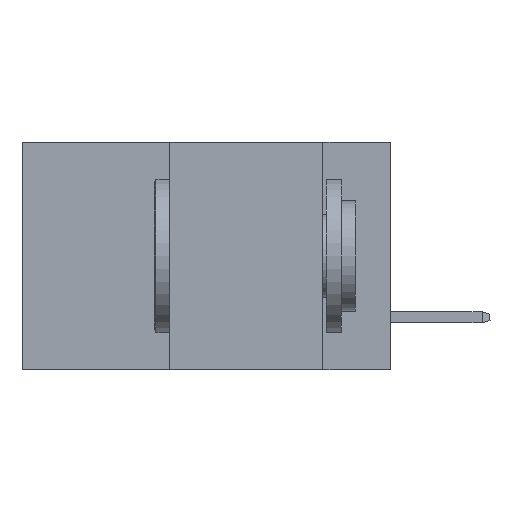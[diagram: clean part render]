
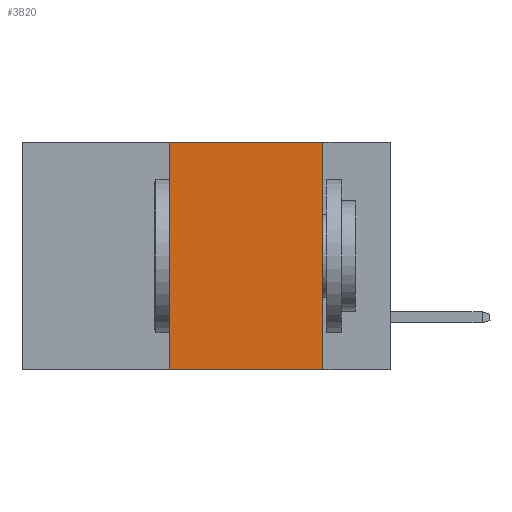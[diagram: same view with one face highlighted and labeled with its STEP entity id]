
A CAD part, left-side view. The second image highlights one B-rep face of the part: STEP entity #3820.
In plain terms, the highlighted planar face has unit normal (-1, 0, 0).
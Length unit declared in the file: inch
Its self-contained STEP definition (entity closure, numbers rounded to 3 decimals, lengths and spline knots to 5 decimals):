
#762 = DIRECTION ( 'NONE',  ( 0., 0., -1. ) ) ;
#984 = LINE ( 'NONE', #3387, #13272 ) ;
#1010 = EDGE_CURVE ( 'NONE', #9239, #12573, #7434, .T. ) ;
#1478 = DIRECTION ( 'NONE',  ( 0., -1., 0. ) ) ;
#2253 = FACE_OUTER_BOUND ( 'NONE', #3483, .T. ) ;
#3256 = ORIENTED_EDGE ( 'NONE', *, *, #9464, .F. ) ;
#3387 = CARTESIAN_POINT ( 'NONE',  ( 0., 0.6, -0.37 ) ) ;
#3483 = EDGE_LOOP ( 'NONE', ( #3256, #3756, #3865, #6334 ) ) ;
#3705 = CARTESIAN_POINT ( 'NONE',  ( 0., 0.11, 0. ) ) ;
#3756 = ORIENTED_EDGE ( 'NONE', *, *, #11149, .F. ) ;
#3820 = ADVANCED_FACE ( 'NONE', ( #2253 ), #4239, .F. ) ;
#3865 = ORIENTED_EDGE ( 'NONE', *, *, #1010, .F. ) ;
#4069 = DIRECTION ( 'NONE',  ( 0., 0., -1. ) ) ;
#4072 = DIRECTION ( 'NONE',  ( 1., 0., 0. ) ) ;
#4223 = CARTESIAN_POINT ( 'NONE',  ( 0., 0.6, 0. ) ) ;
#4239 = PLANE ( 'NONE',  #12794 ) ;
#4615 = VECTOR ( 'NONE', #6443, 39.37008 ) ;
#4671 = CARTESIAN_POINT ( 'NONE',  ( 0., 0.6, 0. ) ) ;
#5571 = LINE ( 'NONE', #4671, #13184 ) ;
#6334 = ORIENTED_EDGE ( 'NONE', *, *, #13311, .T. ) ;
#6443 = DIRECTION ( 'NONE',  ( 0., 0., 1. ) ) ;
#6706 = VERTEX_POINT ( 'NONE', #3705 ) ;
#7434 = LINE ( 'NONE', #9968, #4615 ) ;
#8384 = CARTESIAN_POINT ( 'NONE',  ( 0., 0.11, -0.37 ) ) ;
#9239 = VERTEX_POINT ( 'NONE', #11752 ) ;
#9464 = EDGE_CURVE ( 'NONE', #6706, #11489, #13065, .T. ) ;
#9968 = CARTESIAN_POINT ( 'NONE',  ( 0., 0.36, 0. ) ) ;
#10148 = CARTESIAN_POINT ( 'NONE',  ( 0., 0.11, 0. ) ) ;
#10520 = VECTOR ( 'NONE', #762, 39.37008 ) ;
#11149 = EDGE_CURVE ( 'NONE', #12573, #6706, #5571, .T. ) ;
#11489 = VERTEX_POINT ( 'NONE', #8384 ) ;
#11752 = CARTESIAN_POINT ( 'NONE',  ( 0., 0.36, -0.37 ) ) ;
#12173 = CARTESIAN_POINT ( 'NONE',  ( 0., 0.36, 0. ) ) ;
#12499 = DIRECTION ( 'NONE',  ( 0., -1., 0. ) ) ;
#12573 = VERTEX_POINT ( 'NONE', #12173 ) ;
#12794 = AXIS2_PLACEMENT_3D ( 'NONE', #4223, #4072, #4069 ) ;
#13065 = LINE ( 'NONE', #10148, #10520 ) ;
#13184 = VECTOR ( 'NONE', #1478, 39.37008 ) ;
#13272 = VECTOR ( 'NONE', #12499, 39.37008 ) ;
#13311 = EDGE_CURVE ( 'NONE', #9239, #11489, #984, .T. ) ;
